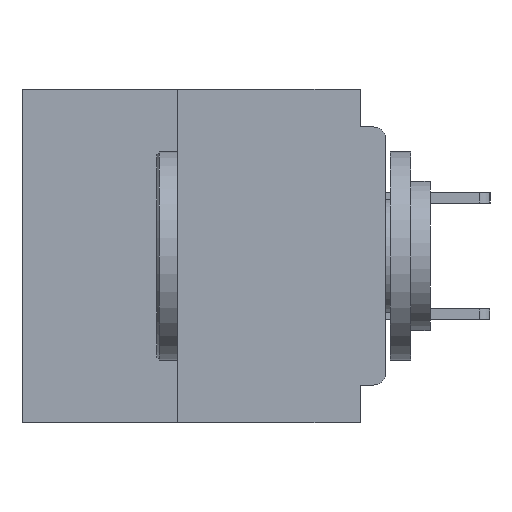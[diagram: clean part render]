
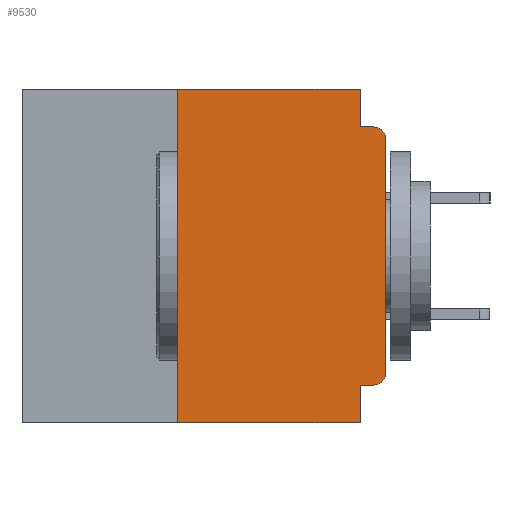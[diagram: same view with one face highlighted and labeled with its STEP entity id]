
A CAD part, left-side view. The second image highlights one B-rep face of the part: STEP entity #9530.
In plain terms, the highlighted planar face has unit normal (-1, 0, 0).
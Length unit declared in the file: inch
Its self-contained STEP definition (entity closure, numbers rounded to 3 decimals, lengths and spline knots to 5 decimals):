
#777 = DIRECTION ( 'NONE',  ( 1., 0., 0. ) ) ;
#1449 = DIRECTION ( 'NONE',  ( 0., 0., 1. ) ) ;
#2345 = EDGE_CURVE ( 'NONE', #32879, #13133, #54261, .T. ) ;
#2730 = CARTESIAN_POINT ( 'NONE',  ( 0., 0.015, -0.06 ) ) ;
#2851 = VECTOR ( 'NONE', #1449, 39.37008 ) ;
#3646 = EDGE_CURVE ( 'NONE', #3659, #50267, #8423, .T. ) ;
#3659 = VERTEX_POINT ( 'NONE', #35126 ) ;
#4956 = ORIENTED_EDGE ( 'NONE', *, *, #46625, .F. ) ;
#5163 = CARTESIAN_POINT ( 'NONE',  ( 0., 0.437, 0. ) ) ;
#6008 = CARTESIAN_POINT ( 'NONE',  ( 0., 0., -0.34 ) ) ;
#7009 = VECTOR ( 'NONE', #34679, 39.37008 ) ;
#7301 = DIRECTION ( 'NONE',  ( 0., 0., -1. ) ) ;
#7755 = VECTOR ( 'NONE', #15144, 39.37008 ) ;
#8410 = LINE ( 'NONE', #40385, #32363 ) ;
#8423 = LINE ( 'NONE', #37331, #7009 ) ;
#9530 = ADVANCED_FACE ( 'NONE', ( #28363 ), #54751, .F. ) ;
#9694 = LINE ( 'NONE', #14156, #20301 ) ;
#9767 = ORIENTED_EDGE ( 'NONE', *, *, #53098, .T. ) ;
#10292 = CARTESIAN_POINT ( 'NONE',  ( 0., 0.031, 0. ) ) ;
#10491 = EDGE_CURVE ( 'NONE', #13133, #20760, #50766, .T. ) ;
#11264 = ORIENTED_EDGE ( 'NONE', *, *, #2345, .T. ) ;
#11789 = EDGE_CURVE ( 'NONE', #3659, #41081, #54230, .T. ) ;
#12790 = CARTESIAN_POINT ( 'NONE',  ( 0., 0.031, -0.355 ) ) ;
#13133 = VERTEX_POINT ( 'NONE', #6008 ) ;
#13438 = VECTOR ( 'NONE', #48727, 39.37008 ) ;
#14156 = CARTESIAN_POINT ( 'NONE',  ( 0., 0., -0.355 ) ) ;
#15144 = DIRECTION ( 'NONE',  ( 0., -1., 0. ) ) ;
#15449 = ORIENTED_EDGE ( 'NONE', *, *, #3646, .F. ) ;
#16876 = ORIENTED_EDGE ( 'NONE', *, *, #28861, .F. ) ;
#17251 = CARTESIAN_POINT ( 'NONE',  ( 0., 0.437, 0. ) ) ;
#17956 = DIRECTION ( 'NONE',  ( 0., 0., -1. ) ) ;
#18506 = ORIENTED_EDGE ( 'NONE', *, *, #11789, .T. ) ;
#18574 = VERTEX_POINT ( 'NONE', #12790 ) ;
#19448 = CARTESIAN_POINT ( 'NONE',  ( 0., 0., 0. ) ) ;
#20301 = VECTOR ( 'NONE', #45665, 39.37008 ) ;
#20463 = AXIS2_PLACEMENT_3D ( 'NONE', #24918, #24725, #24709 ) ;
#20760 = VERTEX_POINT ( 'NONE', #32108 ) ;
#21231 = VERTEX_POINT ( 'NONE', #57610 ) ;
#21964 = ORIENTED_EDGE ( 'NONE', *, *, #47358, .F. ) ;
#23591 = VERTEX_POINT ( 'NONE', #50113 ) ;
#24709 = DIRECTION ( 'NONE',  ( 0., 0., -1. ) ) ;
#24725 = DIRECTION ( 'NONE',  ( -1., 0., 0. ) ) ;
#24918 = CARTESIAN_POINT ( 'NONE',  ( 0., 0.015, -0.34 ) ) ;
#25432 = LINE ( 'NONE', #17251, #13438 ) ;
#26143 = LINE ( 'NONE', #56861, #48672 ) ;
#26916 = ORIENTED_EDGE ( 'NONE', *, *, #31528, .F. ) ;
#28363 = FACE_OUTER_BOUND ( 'NONE', #51640, .T. ) ;
#28861 = EDGE_CURVE ( 'NONE', #32879, #18574, #9694, .T. ) ;
#29730 = LINE ( 'NONE', #10292, #52239 ) ;
#31528 = EDGE_CURVE ( 'NONE', #21231, #47404, #26143, .T. ) ;
#32108 = CARTESIAN_POINT ( 'NONE',  ( 0., 0., -0.06 ) ) ;
#32347 = DIRECTION ( 'NONE',  ( 0., 0., -1. ) ) ;
#32363 = VECTOR ( 'NONE', #17956, 39.37008 ) ;
#32619 = CARTESIAN_POINT ( 'NONE',  ( 0., 0.031, -0.4 ) ) ;
#32879 = VERTEX_POINT ( 'NONE', #44191 ) ;
#34262 = DIRECTION ( 'NONE',  ( -1., 0., 0. ) ) ;
#34446 = DIRECTION ( 'NONE',  ( 0., -1., 0. ) ) ;
#34679 = DIRECTION ( 'NONE',  ( 0., 0., 1. ) ) ;
#35126 = CARTESIAN_POINT ( 'NONE',  ( 0., 0.25, -0.4 ) ) ;
#35580 = ORIENTED_EDGE ( 'NONE', *, *, #50909, .F. ) ;
#36902 = AXIS2_PLACEMENT_3D ( 'NONE', #5163, #777, #32347 ) ;
#37331 = CARTESIAN_POINT ( 'NONE',  ( 0., 0.25, -0.4 ) ) ;
#40385 = CARTESIAN_POINT ( 'NONE',  ( 0., 0.031, -0.4 ) ) ;
#41081 = VERTEX_POINT ( 'NONE', #32619 ) ;
#42127 = CARTESIAN_POINT ( 'NONE',  ( 0., 0.437, -0.4 ) ) ;
#44191 = CARTESIAN_POINT ( 'NONE',  ( 0., 0.015, -0.355 ) ) ;
#45111 = CARTESIAN_POINT ( 'NONE',  ( 0., 0.015, -0.045 ) ) ;
#45665 = DIRECTION ( 'NONE',  ( 0., 1., 0. ) ) ;
#46317 = DIRECTION ( 'NONE',  ( 0., 0., -1. ) ) ;
#46625 = EDGE_CURVE ( 'NONE', #50267, #23591, #25432, .T. ) ;
#47358 = EDGE_CURVE ( 'NONE', #18574, #41081, #8410, .T. ) ;
#47404 = VERTEX_POINT ( 'NONE', #45111 ) ;
#48672 = VECTOR ( 'NONE', #34446, 39.37008 ) ;
#48727 = DIRECTION ( 'NONE',  ( 0., -1., 0. ) ) ;
#50113 = CARTESIAN_POINT ( 'NONE',  ( 0., 0.031, 0. ) ) ;
#50267 = VERTEX_POINT ( 'NONE', #51688 ) ;
#50766 = LINE ( 'NONE', #19448, #2851 ) ;
#50909 = EDGE_CURVE ( 'NONE', #23591, #21231, #29730, .T. ) ;
#51640 = EDGE_LOOP ( 'NONE', ( #55332, #9767, #26916, #35580, #4956, #15449, #18506, #21964, #16876, #11264 ) ) ;
#51688 = CARTESIAN_POINT ( 'NONE',  ( 0., 0.25, 0. ) ) ;
#52239 = VECTOR ( 'NONE', #46317, 39.37008 ) ;
#53098 = EDGE_CURVE ( 'NONE', #20760, #47404, #54745, .T. ) ;
#54230 = LINE ( 'NONE', #42127, #7755 ) ;
#54261 = CIRCLE ( 'NONE', #20463, 0.015 ) ;
#54745 = CIRCLE ( 'NONE', #57347, 0.015 ) ;
#54751 = PLANE ( 'NONE',  #36902 ) ;
#55332 = ORIENTED_EDGE ( 'NONE', *, *, #10491, .T. ) ;
#56861 = CARTESIAN_POINT ( 'NONE',  ( 0., 0., -0.045 ) ) ;
#57347 = AXIS2_PLACEMENT_3D ( 'NONE', #2730, #34262, #7301 ) ;
#57610 = CARTESIAN_POINT ( 'NONE',  ( 0., 0.031, -0.045 ) ) ;
